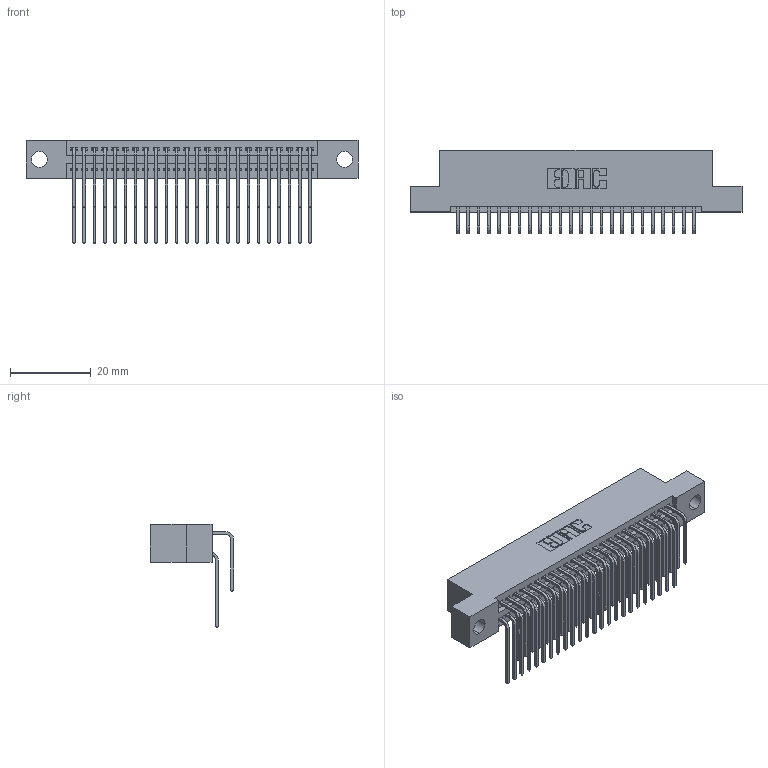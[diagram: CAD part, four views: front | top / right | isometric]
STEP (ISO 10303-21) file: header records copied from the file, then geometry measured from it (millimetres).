
FILE_DESCRIPTION (( 'STEP AP203' ), '1' );
FILE_NAME ('395-048-559-204.STEP', '2018-11-19T23:47:47', ( '' ), ( '' ), 'SwSTEP 2.0', 'SolidWorks 2016', '' );
FILE_SCHEMA (( 'CONFIG_CONTROL_DESIGN' ));
Length unit declared in the file: inch
Products named in the file (4): 395-048-559-204; 345 Part_Flush Mounting Lugs - 0.156 Dia-TH; 345-292-001_558 559 Tail - 1; 345-292-001_559 Tail - 2
Assembly tree (49 placements, depth 2):
  395-048-559-204
    345 Part_Flush Mounting Lugs - 0.156 Dia-TH
    345-292-001_558 559 Tail - 1  x24
    345-292-001_559 Tail - 2  x24
Bounding box: 82.17 x 20.56 x 25.53 mm (x, y, z)
Volume: 8003.9 mm3; surface area: 12599.8 mm2
Topology: 49 solids, 49 shells, 2622 faces, 7781 edges, 5122 vertices
Faces by surface type: plane 1760, cylinder 862
Entity records: 22909 total; most frequent: CARTESIAN_POINT 3903, ORIENTED_EDGE 3786, DIRECTION 3437, EDGE_CURVE 1893, VECTOR 1625, LINE 1625, VERTEX_POINT 1258, AXIS2_PLACEMENT_3D 906
